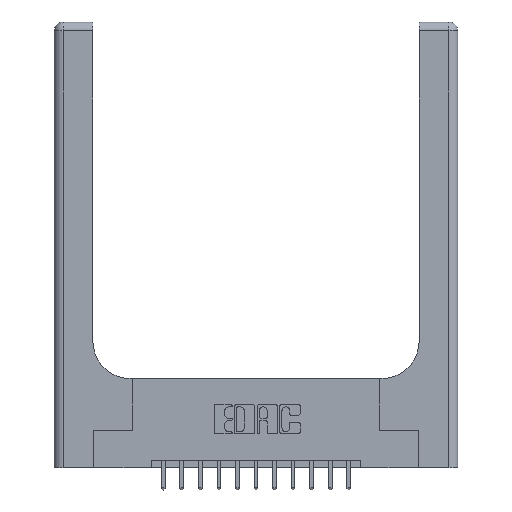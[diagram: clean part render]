
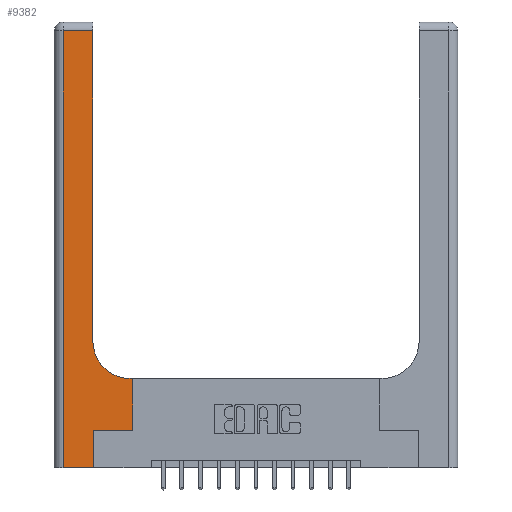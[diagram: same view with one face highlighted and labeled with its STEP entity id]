
A CAD part, top view. The second image highlights one B-rep face of the part: STEP entity #9382.
In plain terms, the highlighted planar face has unit normal (0, 0, 1).
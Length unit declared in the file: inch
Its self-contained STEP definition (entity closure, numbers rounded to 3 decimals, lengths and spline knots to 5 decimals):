
#658 = DIRECTION ( 'NONE',  ( 0., 1., 0. ) ) ;
#714 = CARTESIAN_POINT ( 'NONE',  ( 0.26, 3., 0.37 ) ) ;
#1340 = LINE ( 'NONE', #2519, #13181 ) ;
#1345 = CARTESIAN_POINT ( 'NONE',  ( 0., 3., 0.37 ) ) ;
#1855 = VECTOR ( 'NONE', #658, 39.37008 ) ;
#2098 = LINE ( 'NONE', #14559, #12145 ) ;
#2519 = CARTESIAN_POINT ( 'NONE',  ( 0.26, 0.6, 0.37 ) ) ;
#2590 = VECTOR ( 'NONE', #16094, 39.37008 ) ;
#2847 = VERTEX_POINT ( 'NONE', #8124 ) ;
#2881 = ORIENTED_EDGE ( 'NONE', *, *, #12373, .T. ) ;
#3182 = EDGE_CURVE ( 'NONE', #12325, #15312, #10585, .T. ) ;
#3309 = DIRECTION ( 'NONE',  ( 0., -1., 0. ) ) ;
#3324 = EDGE_CURVE ( 'NONE', #12620, #9478, #11962, .T. ) ;
#3365 = VECTOR ( 'NONE', #7793, 39.37008 ) ;
#3753 = VECTOR ( 'NONE', #3309, 39.37008 ) ;
#3784 = CARTESIAN_POINT ( 'NONE',  ( 0.265, 0.25, 0.37 ) ) ;
#3821 = ORIENTED_EDGE ( 'NONE', *, *, #11808, .T. ) ;
#4496 = FACE_OUTER_BOUND ( 'NONE', #12432, .T. ) ;
#4504 = ORIENTED_EDGE ( 'NONE', *, *, #11540, .T. ) ;
#4964 = LINE ( 'NONE', #7739, #3365 ) ;
#5189 = DIRECTION ( 'NONE',  ( 0., 0., -1. ) ) ;
#5304 = LINE ( 'NONE', #9777, #8718 ) ;
#5443 = DIRECTION ( 'NONE',  ( 1., 0., 0. ) ) ;
#5482 = ORIENTED_EDGE ( 'NONE', *, *, #3182, .T. ) ;
#5940 = VECTOR ( 'NONE', #7615, 39.37008 ) ;
#6008 = ORIENTED_EDGE ( 'NONE', *, *, #8528, .T. ) ;
#6637 = LINE ( 'NONE', #714, #1855 ) ;
#7076 = VERTEX_POINT ( 'NONE', #12818 ) ;
#7203 = LINE ( 'NONE', #15006, #2590 ) ;
#7615 = DIRECTION ( 'NONE',  ( 0., 1., 0. ) ) ;
#7739 = CARTESIAN_POINT ( 'NONE',  ( 0.528, 0.25, 0.37 ) ) ;
#7793 = DIRECTION ( 'NONE',  ( 0., 1., 0. ) ) ;
#7808 = AXIS2_PLACEMENT_3D ( 'NONE', #14447, #15798, #10610 ) ;
#8097 = VERTEX_POINT ( 'NONE', #14119 ) ;
#8124 = CARTESIAN_POINT ( 'NONE',  ( 0.528, 0.25, 0.37 ) ) ;
#8528 = EDGE_CURVE ( 'NONE', #15312, #12620, #5304, .T. ) ;
#8539 = AXIS2_PLACEMENT_3D ( 'NONE', #1345, #5189, #15360 ) ;
#8570 = CARTESIAN_POINT ( 'NONE',  ( 0.265, 0., 0.37 ) ) ;
#8718 = VECTOR ( 'NONE', #15985, 39.37008 ) ;
#9382 = ADVANCED_FACE ( 'NONE', ( #4496 ), #10108, .F. ) ;
#9478 = VERTEX_POINT ( 'NONE', #3784 ) ;
#9711 = CARTESIAN_POINT ( 'NONE',  ( 0.06, 3., 0.37 ) ) ;
#9777 = CARTESIAN_POINT ( 'NONE',  ( 0., 0., 0.37 ) ) ;
#10108 = PLANE ( 'NONE',  #8539 ) ;
#10585 = LINE ( 'NONE', #9711, #3753 ) ;
#10610 = DIRECTION ( 'NONE',  ( 1., 0., 0. ) ) ;
#10755 = EDGE_CURVE ( 'NONE', #14453, #7076, #6637, .T. ) ;
#10965 = CARTESIAN_POINT ( 'NONE',  ( 0.06, 0., 0.37 ) ) ;
#11315 = EDGE_CURVE ( 'NONE', #7076, #12325, #7203, .T. ) ;
#11540 = EDGE_CURVE ( 'NONE', #8097, #14453, #11995, .T. ) ;
#11808 = EDGE_CURVE ( 'NONE', #12993, #8097, #1340, .T. ) ;
#11962 = LINE ( 'NONE', #8570, #5940 ) ;
#11995 = CIRCLE ( 'NONE', #7808, 0.25 ) ;
#12145 = VECTOR ( 'NONE', #5443, 39.37008 ) ;
#12325 = VERTEX_POINT ( 'NONE', #16388 ) ;
#12373 = EDGE_CURVE ( 'NONE', #2847, #12993, #4964, .T. ) ;
#12432 = EDGE_LOOP ( 'NONE', ( #13059, #12862, #5482, #6008, #13678, #15673, #2881, #3821, #4504 ) ) ;
#12620 = VERTEX_POINT ( 'NONE', #13221 ) ;
#12688 = DIRECTION ( 'NONE',  ( -1., 0., 0. ) ) ;
#12818 = CARTESIAN_POINT ( 'NONE',  ( 0.26, 2.94, 0.37 ) ) ;
#12862 = ORIENTED_EDGE ( 'NONE', *, *, #11315, .T. ) ;
#12993 = VERTEX_POINT ( 'NONE', #13262 ) ;
#13059 = ORIENTED_EDGE ( 'NONE', *, *, #10755, .T. ) ;
#13173 = EDGE_CURVE ( 'NONE', #9478, #2847, #2098, .T. ) ;
#13181 = VECTOR ( 'NONE', #12688, 39.37008 ) ;
#13221 = CARTESIAN_POINT ( 'NONE',  ( 0.265, 0., 0.37 ) ) ;
#13262 = CARTESIAN_POINT ( 'NONE',  ( 0.528, 0.6, 0.37 ) ) ;
#13678 = ORIENTED_EDGE ( 'NONE', *, *, #3324, .T. ) ;
#14119 = CARTESIAN_POINT ( 'NONE',  ( 0.51, 0.6, 0.37 ) ) ;
#14447 = CARTESIAN_POINT ( 'NONE',  ( 0.51, 0.85, 0.37 ) ) ;
#14453 = VERTEX_POINT ( 'NONE', #15707 ) ;
#14559 = CARTESIAN_POINT ( 'NONE',  ( 0.265, 0.25, 0.37 ) ) ;
#15006 = CARTESIAN_POINT ( 'NONE',  ( 0., 2.94, 0.37 ) ) ;
#15312 = VERTEX_POINT ( 'NONE', #10965 ) ;
#15360 = DIRECTION ( 'NONE',  ( -1., 0., 0. ) ) ;
#15673 = ORIENTED_EDGE ( 'NONE', *, *, #13173, .T. ) ;
#15707 = CARTESIAN_POINT ( 'NONE',  ( 0.26, 0.85, 0.37 ) ) ;
#15798 = DIRECTION ( 'NONE',  ( 0., 0., -1. ) ) ;
#15985 = DIRECTION ( 'NONE',  ( 1., 0., 0. ) ) ;
#16094 = DIRECTION ( 'NONE',  ( -1., 0., 0. ) ) ;
#16388 = CARTESIAN_POINT ( 'NONE',  ( 0.06, 2.94, 0.37 ) ) ;
